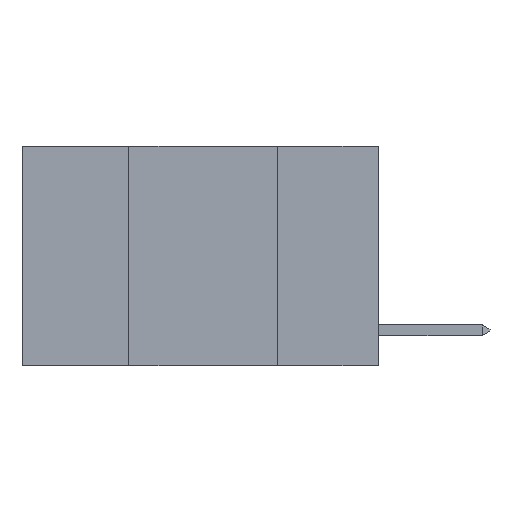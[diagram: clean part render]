
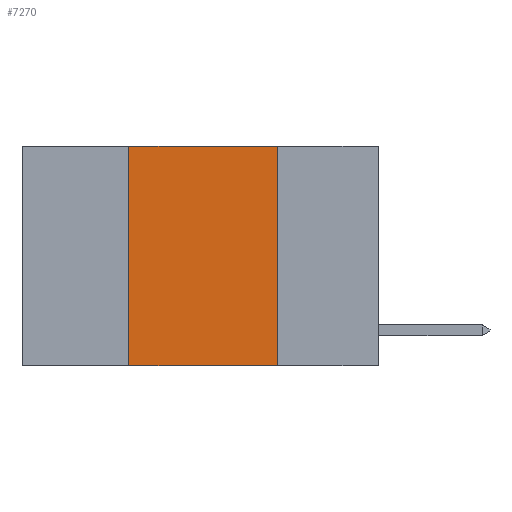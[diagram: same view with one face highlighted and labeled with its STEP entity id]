
A CAD part, left-side view. The second image highlights one B-rep face of the part: STEP entity #7270.
In plain terms, the highlighted planar face has unit normal (-1, 0, 0).
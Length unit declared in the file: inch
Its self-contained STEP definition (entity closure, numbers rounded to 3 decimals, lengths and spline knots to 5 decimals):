
#1137 = DIRECTION ( 'NONE',  ( 0., -1., 0. ) ) ;
#1220 = VERTEX_POINT ( 'NONE', #14730 ) ;
#1851 = EDGE_LOOP ( 'NONE', ( #11162, #12566, #14269, #14330 ) ) ;
#2029 = EDGE_CURVE ( 'NONE', #13962, #1220, #13373, .T. ) ;
#2082 = AXIS2_PLACEMENT_3D ( 'NONE', #8741, #9911, #2373 ) ;
#2273 = EDGE_CURVE ( 'NONE', #1220, #5207, #6216, .T. ) ;
#2373 = DIRECTION ( 'NONE',  ( 0., 0., -1. ) ) ;
#3020 = VECTOR ( 'NONE', #1137, 39.37008 ) ;
#3134 = LINE ( 'NONE', #15632, #15685 ) ;
#3743 = DIRECTION ( 'NONE',  ( 0., 0., 1. ) ) ;
#4501 = EDGE_CURVE ( 'NONE', #12046, #5207, #3134, .T. ) ;
#4703 = VECTOR ( 'NONE', #3743, 39.37008 ) ;
#4786 = EDGE_CURVE ( 'NONE', #12046, #13962, #14680, .T. ) ;
#5207 = VERTEX_POINT ( 'NONE', #13429 ) ;
#6216 = LINE ( 'NONE', #9267, #15761 ) ;
#7079 = CARTESIAN_POINT ( 'NONE',  ( 0., 0.42, -0.37 ) ) ;
#7270 = ADVANCED_FACE ( 'NONE', ( #15631 ), #7448, .F. ) ;
#7448 = PLANE ( 'NONE',  #2082 ) ;
#8741 = CARTESIAN_POINT ( 'NONE',  ( 0., 0.6, 0. ) ) ;
#9267 = CARTESIAN_POINT ( 'NONE',  ( 0., 0.17, 0. ) ) ;
#9677 = CARTESIAN_POINT ( 'NONE',  ( 0., 0.42, 0. ) ) ;
#9911 = DIRECTION ( 'NONE',  ( 1., 0., 0. ) ) ;
#10446 = DIRECTION ( 'NONE',  ( 0., 0., -1. ) ) ;
#10631 = DIRECTION ( 'NONE',  ( 0., -1., 0. ) ) ;
#11162 = ORIENTED_EDGE ( 'NONE', *, *, #2273, .F. ) ;
#11202 = CARTESIAN_POINT ( 'NONE',  ( 0., 0.42, 0. ) ) ;
#12046 = VERTEX_POINT ( 'NONE', #7079 ) ;
#12389 = CARTESIAN_POINT ( 'NONE',  ( 0., 0.6, 0. ) ) ;
#12566 = ORIENTED_EDGE ( 'NONE', *, *, #2029, .F. ) ;
#13373 = LINE ( 'NONE', #12389, #3020 ) ;
#13429 = CARTESIAN_POINT ( 'NONE',  ( 0., 0.17, -0.37 ) ) ;
#13962 = VERTEX_POINT ( 'NONE', #9677 ) ;
#14269 = ORIENTED_EDGE ( 'NONE', *, *, #4786, .F. ) ;
#14330 = ORIENTED_EDGE ( 'NONE', *, *, #4501, .T. ) ;
#14680 = LINE ( 'NONE', #11202, #4703 ) ;
#14730 = CARTESIAN_POINT ( 'NONE',  ( 0., 0.17, 0. ) ) ;
#15631 = FACE_OUTER_BOUND ( 'NONE', #1851, .T. ) ;
#15632 = CARTESIAN_POINT ( 'NONE',  ( 0., 0.6, -0.37 ) ) ;
#15685 = VECTOR ( 'NONE', #10631, 39.37008 ) ;
#15761 = VECTOR ( 'NONE', #10446, 39.37008 ) ;
